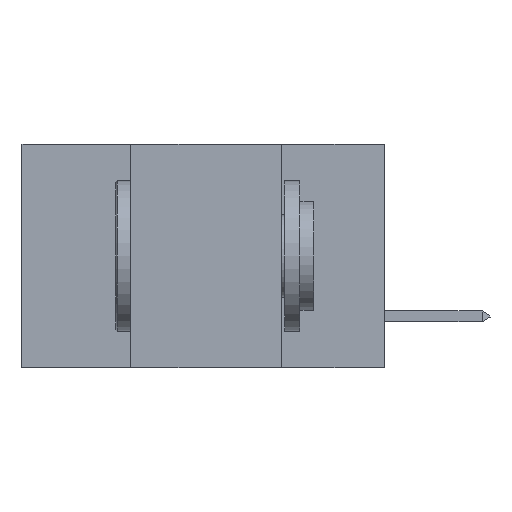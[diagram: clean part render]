
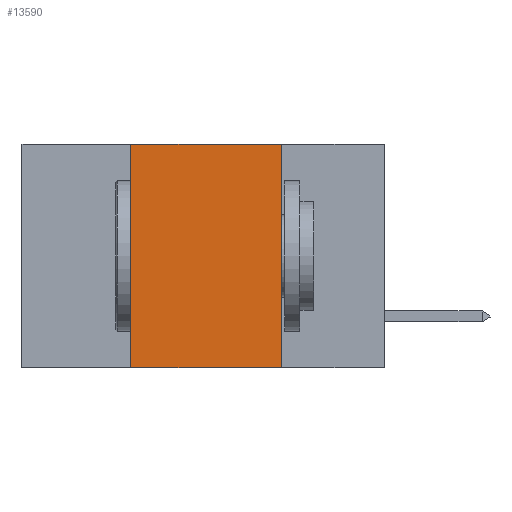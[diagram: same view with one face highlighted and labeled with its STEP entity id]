
A CAD part, left-side view. The second image highlights one B-rep face of the part: STEP entity #13590.
In plain terms, the highlighted planar face has unit normal (-1, 0, 0).
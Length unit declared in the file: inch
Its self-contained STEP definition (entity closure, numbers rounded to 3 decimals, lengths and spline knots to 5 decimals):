
#354 = VERTEX_POINT ( 'NONE', #7775 ) ;
#1029 = EDGE_LOOP ( 'NONE', ( #14658, #27124, #11812, #28175 ) ) ;
#1298 = PLANE ( 'NONE',  #10203 ) ;
#3057 = CARTESIAN_POINT ( 'NONE',  ( 0., 0.6, -0.37 ) ) ;
#3591 = CARTESIAN_POINT ( 'NONE',  ( 0., 0.6, 0. ) ) ;
#5341 = DIRECTION ( 'NONE',  ( 0., -1., 0. ) ) ;
#5952 = EDGE_CURVE ( 'NONE', #13323, #20994, #13104, .T. ) ;
#5964 = DIRECTION ( 'NONE',  ( 1., 0., 0. ) ) ;
#6745 = EDGE_CURVE ( 'NONE', #20218, #354, #21633, .T. ) ;
#7443 = VECTOR ( 'NONE', #27023, 39.37008 ) ;
#7775 = CARTESIAN_POINT ( 'NONE',  ( 0., 0.17, -0.37 ) ) ;
#8600 = CARTESIAN_POINT ( 'NONE',  ( 0., 0.6, 0. ) ) ;
#10203 = AXIS2_PLACEMENT_3D ( 'NONE', #3591, #5964, #19606 ) ;
#11812 = ORIENTED_EDGE ( 'NONE', *, *, #5952, .F. ) ;
#13104 = LINE ( 'NONE', #22126, #15593 ) ;
#13323 = VERTEX_POINT ( 'NONE', #13393 ) ;
#13393 = CARTESIAN_POINT ( 'NONE',  ( 0., 0.42, -0.37 ) ) ;
#13590 = ADVANCED_FACE ( 'NONE', ( #27624 ), #1298, .F. ) ;
#14630 = CARTESIAN_POINT ( 'NONE',  ( 0., 0.17, 0. ) ) ;
#14658 = ORIENTED_EDGE ( 'NONE', *, *, #6745, .F. ) ;
#15562 = VECTOR ( 'NONE', #28874, 39.37008 ) ;
#15593 = VECTOR ( 'NONE', #19833, 39.37008 ) ;
#17883 = CARTESIAN_POINT ( 'NONE',  ( 0., 0.17, 0. ) ) ;
#19606 = DIRECTION ( 'NONE',  ( 0., 0., -1. ) ) ;
#19833 = DIRECTION ( 'NONE',  ( 0., 0., 1. ) ) ;
#20218 = VERTEX_POINT ( 'NONE', #14630 ) ;
#20994 = VERTEX_POINT ( 'NONE', #28945 ) ;
#21633 = LINE ( 'NONE', #17883, #15562 ) ;
#21907 = LINE ( 'NONE', #3057, #28964 ) ;
#22126 = CARTESIAN_POINT ( 'NONE',  ( 0., 0.42, 0. ) ) ;
#22708 = LINE ( 'NONE', #8600, #7443 ) ;
#22996 = EDGE_CURVE ( 'NONE', #13323, #354, #21907, .T. ) ;
#27023 = DIRECTION ( 'NONE',  ( 0., -1., 0. ) ) ;
#27124 = ORIENTED_EDGE ( 'NONE', *, *, #29015, .F. ) ;
#27624 = FACE_OUTER_BOUND ( 'NONE', #1029, .T. ) ;
#28175 = ORIENTED_EDGE ( 'NONE', *, *, #22996, .T. ) ;
#28874 = DIRECTION ( 'NONE',  ( 0., 0., -1. ) ) ;
#28945 = CARTESIAN_POINT ( 'NONE',  ( 0., 0.42, 0. ) ) ;
#28964 = VECTOR ( 'NONE', #5341, 39.37008 ) ;
#29015 = EDGE_CURVE ( 'NONE', #20994, #20218, #22708, .T. ) ;
